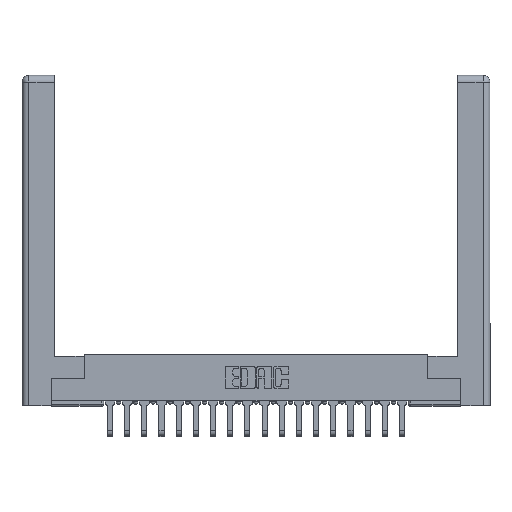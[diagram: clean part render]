
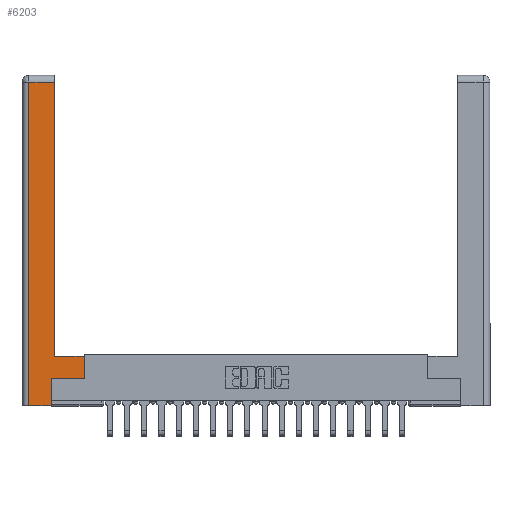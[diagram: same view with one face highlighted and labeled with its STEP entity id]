
A CAD part, top view. The second image highlights one B-rep face of the part: STEP entity #6203.
In plain terms, the highlighted planar face has unit normal (0, 0, 1).
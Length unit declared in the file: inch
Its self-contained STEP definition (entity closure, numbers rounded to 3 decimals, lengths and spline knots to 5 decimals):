
#890 = VECTOR ( 'NONE', #12577, 39.37008 ) ;
#895 = EDGE_CURVE ( 'NONE', #15988, #17189, #13591, .T. ) ;
#1574 = LINE ( 'NONE', #11622, #13542 ) ;
#1619 = VECTOR ( 'NONE', #19306, 39.37008 ) ;
#1621 = EDGE_CURVE ( 'NONE', #8978, #15988, #4145, .T. ) ;
#2181 = VERTEX_POINT ( 'NONE', #7354 ) ;
#2182 = FACE_OUTER_BOUND ( 'NONE', #6094, .T. ) ;
#2228 = DIRECTION ( 'NONE',  ( -1., 0., 0. ) ) ;
#2544 = VECTOR ( 'NONE', #6804, 39.37008 ) ;
#3052 = LINE ( 'NONE', #9827, #2544 ) ;
#3205 = PLANE ( 'NONE',  #10730 ) ;
#3221 = ORIENTED_EDGE ( 'NONE', *, *, #1621, .T. ) ;
#3835 = ORIENTED_EDGE ( 'NONE', *, *, #895, .T. ) ;
#4145 = LINE ( 'NONE', #13881, #7712 ) ;
#4163 = DIRECTION ( 'NONE',  ( 0., 1., 0. ) ) ;
#4852 = CARTESIAN_POINT ( 'NONE',  ( 0., 0., 0. ) ) ;
#4908 = CARTESIAN_POINT ( 'NONE',  ( 0.295, 0.45, 0. ) ) ;
#5308 = LINE ( 'NONE', #17326, #20332 ) ;
#5841 = VERTEX_POINT ( 'NONE', #20023 ) ;
#6094 = EDGE_LOOP ( 'NONE', ( #18068, #9998, #16161, #15499, #3221, #3835, #9423, #12270 ) ) ;
#6105 = VERTEX_POINT ( 'NONE', #19129 ) ;
#6203 = ADVANCED_FACE ( 'NONE', ( #2182 ), #3205, .F. ) ;
#6804 = DIRECTION ( 'NONE',  ( 0., 1., 0. ) ) ;
#7354 = CARTESIAN_POINT ( 'NONE',  ( 0.0615, 0., 0. ) ) ;
#7489 = LINE ( 'NONE', #11999, #15618 ) ;
#7578 = CARTESIAN_POINT ( 'NONE',  ( 0.565, 0.45, 0. ) ) ;
#7712 = VECTOR ( 'NONE', #4163, 39.37008 ) ;
#7945 = CARTESIAN_POINT ( 'NONE',  ( 0.0615, 0., 0. ) ) ;
#8274 = EDGE_CURVE ( 'NONE', #13299, #6105, #3052, .T. ) ;
#8319 = DIRECTION ( 'NONE',  ( -1., 0., 0. ) ) ;
#8495 = VECTOR ( 'NONE', #12715, 39.37008 ) ;
#8978 = VERTEX_POINT ( 'NONE', #16358 ) ;
#9015 = CARTESIAN_POINT ( 'NONE',  ( 0.565, 0.245, 0. ) ) ;
#9143 = CARTESIAN_POINT ( 'NONE',  ( 0.565, 0.245, 0. ) ) ;
#9266 = LINE ( 'NONE', #7945, #1619 ) ;
#9423 = ORIENTED_EDGE ( 'NONE', *, *, #10837, .T. ) ;
#9827 = CARTESIAN_POINT ( 'NONE',  ( 0.295, 3., 0. ) ) ;
#9998 = ORIENTED_EDGE ( 'NONE', *, *, #14294, .T. ) ;
#10730 = AXIS2_PLACEMENT_3D ( 'NONE', #4852, #11543, #8319 ) ;
#10837 = EDGE_CURVE ( 'NONE', #17189, #16727, #18223, .T. ) ;
#11543 = DIRECTION ( 'NONE',  ( 0., 0., -1. ) ) ;
#11622 = CARTESIAN_POINT ( 'NONE',  ( 0.295, 0.45, 0. ) ) ;
#11999 = CARTESIAN_POINT ( 'NONE',  ( 0.0615, 2.94, 0. ) ) ;
#12270 = ORIENTED_EDGE ( 'NONE', *, *, #14616, .T. ) ;
#12577 = DIRECTION ( 'NONE',  ( 0., 1., 0. ) ) ;
#12715 = DIRECTION ( 'NONE',  ( 1., 0., 0. ) ) ;
#13299 = VERTEX_POINT ( 'NONE', #4908 ) ;
#13542 = VECTOR ( 'NONE', #17922, 39.37008 ) ;
#13591 = LINE ( 'NONE', #9015, #8495 ) ;
#13881 = CARTESIAN_POINT ( 'NONE',  ( 0.265, 0.245, 0. ) ) ;
#13920 = EDGE_CURVE ( 'NONE', #5841, #2181, #9266, .T. ) ;
#14244 = DIRECTION ( 'NONE',  ( 1., 0., 0. ) ) ;
#14294 = EDGE_CURVE ( 'NONE', #6105, #5841, #7489, .T. ) ;
#14616 = EDGE_CURVE ( 'NONE', #16727, #13299, #1574, .T. ) ;
#15499 = ORIENTED_EDGE ( 'NONE', *, *, #17225, .T. ) ;
#15618 = VECTOR ( 'NONE', #2228, 39.37008 ) ;
#15988 = VERTEX_POINT ( 'NONE', #17502 ) ;
#16124 = CARTESIAN_POINT ( 'NONE',  ( 0.565, 0.45, 0. ) ) ;
#16161 = ORIENTED_EDGE ( 'NONE', *, *, #13920, .T. ) ;
#16358 = CARTESIAN_POINT ( 'NONE',  ( 0.265, 0., 0. ) ) ;
#16727 = VERTEX_POINT ( 'NONE', #16124 ) ;
#17189 = VERTEX_POINT ( 'NONE', #9143 ) ;
#17225 = EDGE_CURVE ( 'NONE', #2181, #8978, #5308, .T. ) ;
#17326 = CARTESIAN_POINT ( 'NONE',  ( 0.265, 0., 0. ) ) ;
#17502 = CARTESIAN_POINT ( 'NONE',  ( 0.265, 0.245, 0. ) ) ;
#17922 = DIRECTION ( 'NONE',  ( -1., 0., 0. ) ) ;
#18068 = ORIENTED_EDGE ( 'NONE', *, *, #8274, .T. ) ;
#18223 = LINE ( 'NONE', #7578, #890 ) ;
#19129 = CARTESIAN_POINT ( 'NONE',  ( 0.295, 2.94, 0. ) ) ;
#19306 = DIRECTION ( 'NONE',  ( 0., -1., 0. ) ) ;
#20023 = CARTESIAN_POINT ( 'NONE',  ( 0.0615, 2.94, 0. ) ) ;
#20332 = VECTOR ( 'NONE', #14244, 39.37008 ) ;
